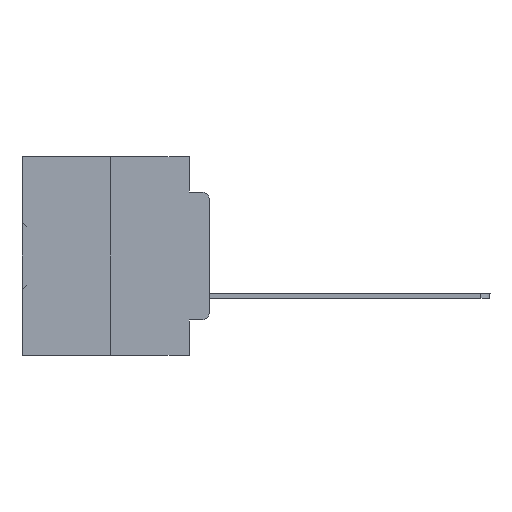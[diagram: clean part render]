
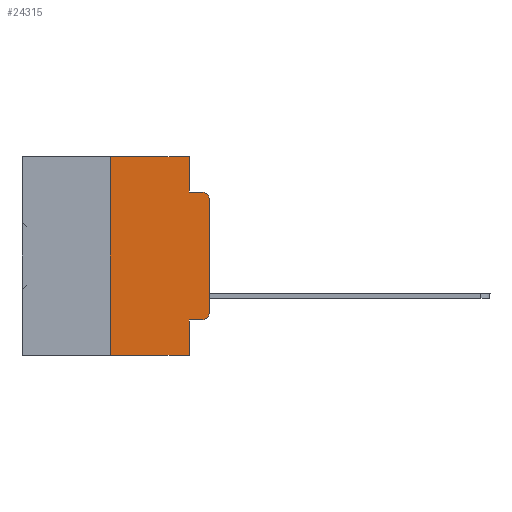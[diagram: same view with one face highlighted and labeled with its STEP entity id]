
A CAD part, left-side view. The second image highlights one B-rep face of the part: STEP entity #24315.
In plain terms, the highlighted planar face has unit normal (-1, 0, 0).
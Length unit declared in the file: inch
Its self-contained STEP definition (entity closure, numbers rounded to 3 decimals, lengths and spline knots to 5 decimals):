
#2049 = LINE ( 'NONE', #13512, #25547 ) ;
#2791 = VERTEX_POINT ( 'NONE', #32330 ) ;
#2859 = VERTEX_POINT ( 'NONE', #7158 ) ;
#3411 = EDGE_CURVE ( 'NONE', #18733, #25055, #25482, .T. ) ;
#3481 = ORIENTED_EDGE ( 'NONE', *, *, #14463, .T. ) ;
#5151 = DIRECTION ( 'NONE',  ( -1., 0., 0. ) ) ;
#5340 = VERTEX_POINT ( 'NONE', #20381 ) ;
#5866 = AXIS2_PLACEMENT_3D ( 'NONE', #30875, #5151, #28058 ) ;
#6440 = ORIENTED_EDGE ( 'NONE', *, *, #6719, .F. ) ;
#6719 = EDGE_CURVE ( 'NONE', #18733, #5340, #20243, .T. ) ;
#6981 = DIRECTION ( 'NONE',  ( 0., 0., -1. ) ) ;
#7158 = CARTESIAN_POINT ( 'NONE',  ( 0., 0.02, -0.0885 ) ) ;
#7283 = VECTOR ( 'NONE', #11411, 39.37008 ) ;
#7359 = CARTESIAN_POINT ( 'NONE',  ( 0., 0.02, -0.1085 ) ) ;
#7740 = ORIENTED_EDGE ( 'NONE', *, *, #14694, .T. ) ;
#8896 = ORIENTED_EDGE ( 'NONE', *, *, #27386, .F. ) ;
#9065 = VECTOR ( 'NONE', #19751, 39.37008 ) ;
#9411 = CARTESIAN_POINT ( 'NONE',  ( 0., 0., -0.3915 ) ) ;
#9613 = CARTESIAN_POINT ( 'NONE',  ( 0., 0.473, 0. ) ) ;
#9690 = LINE ( 'NONE', #21133, #35719 ) ;
#10529 = CIRCLE ( 'NONE', #30297, 0.02 ) ;
#10641 = EDGE_CURVE ( 'NONE', #10848, #15091, #24559, .T. ) ;
#10848 = VERTEX_POINT ( 'NONE', #17407 ) ;
#11054 = EDGE_CURVE ( 'NONE', #5340, #10848, #9690, .T. ) ;
#11411 = DIRECTION ( 'NONE',  ( 0., 0., 1. ) ) ;
#12309 = LINE ( 'NONE', #26766, #20250 ) ;
#12529 = CARTESIAN_POINT ( 'NONE',  ( 0., 0.25, -0.5 ) ) ;
#13048 = VECTOR ( 'NONE', #21058, 39.37008 ) ;
#13512 = CARTESIAN_POINT ( 'NONE',  ( 0., 0.051, -0.4115 ) ) ;
#13858 = ORIENTED_EDGE ( 'NONE', *, *, #3411, .T. ) ;
#14463 = EDGE_CURVE ( 'NONE', #37064, #36121, #12309, .T. ) ;
#14694 = EDGE_CURVE ( 'NONE', #17831, #37064, #20853, .T. ) ;
#15091 = VERTEX_POINT ( 'NONE', #19385 ) ;
#15316 = DIRECTION ( 'NONE',  ( 0., 0., 1. ) ) ;
#15439 = CARTESIAN_POINT ( 'NONE',  ( 0., 0.051, 0. ) ) ;
#16123 = DIRECTION ( 'NONE',  ( 0., 0., -1. ) ) ;
#17407 = CARTESIAN_POINT ( 'NONE',  ( 0., 0.051, 0. ) ) ;
#17831 = VERTEX_POINT ( 'NONE', #26313 ) ;
#18733 = VERTEX_POINT ( 'NONE', #12529 ) ;
#18930 = CARTESIAN_POINT ( 'NONE',  ( 0., 0.051, 0. ) ) ;
#19274 = EDGE_CURVE ( 'NONE', #15091, #2859, #32780, .T. ) ;
#19385 = CARTESIAN_POINT ( 'NONE',  ( 0., 0.051, -0.0885 ) ) ;
#19563 = CARTESIAN_POINT ( 'NONE',  ( 0., 0.051, -0.0885 ) ) ;
#19751 = DIRECTION ( 'NONE',  ( 0., -1., 0. ) ) ;
#19873 = CARTESIAN_POINT ( 'NONE',  ( 0., 0.25, 0. ) ) ;
#20198 = CARTESIAN_POINT ( 'NONE',  ( 0., 0.051, -0.5 ) ) ;
#20243 = LINE ( 'NONE', #19873, #7283 ) ;
#20250 = VECTOR ( 'NONE', #15316, 39.37008 ) ;
#20381 = CARTESIAN_POINT ( 'NONE',  ( 0., 0.25, 0. ) ) ;
#20853 = CIRCLE ( 'NONE', #5866, 0.02 ) ;
#21058 = DIRECTION ( 'NONE',  ( 0., 0., -1. ) ) ;
#21133 = CARTESIAN_POINT ( 'NONE',  ( 0., 0.473, 0. ) ) ;
#21308 = VECTOR ( 'NONE', #16123, 39.37008 ) ;
#22867 = DIRECTION ( 'NONE',  ( 0., -1., 0. ) ) ;
#22950 = ORIENTED_EDGE ( 'NONE', *, *, #11054, .F. ) ;
#24072 = ORIENTED_EDGE ( 'NONE', *, *, #33189, .T. ) ;
#24238 = PLANE ( 'NONE',  #33860 ) ;
#24240 = DIRECTION ( 'NONE',  ( -1., 0., 0. ) ) ;
#24315 = ADVANCED_FACE ( 'NONE', ( #35910 ), #24238, .F. ) ;
#24559 = LINE ( 'NONE', #18930, #21308 ) ;
#25055 = VERTEX_POINT ( 'NONE', #20198 ) ;
#25126 = DIRECTION ( 'NONE',  ( 0., -1., 0. ) ) ;
#25482 = LINE ( 'NONE', #28486, #34034 ) ;
#25547 = VECTOR ( 'NONE', #22867, 39.37008 ) ;
#26313 = CARTESIAN_POINT ( 'NONE',  ( 0., 0.02, -0.4115 ) ) ;
#26394 = CARTESIAN_POINT ( 'NONE',  ( 0., 0., -0.1085 ) ) ;
#26766 = CARTESIAN_POINT ( 'NONE',  ( 0., 0., 0. ) ) ;
#27329 = DIRECTION ( 'NONE',  ( 0., -1., 0. ) ) ;
#27386 = EDGE_CURVE ( 'NONE', #2791, #25055, #29332, .T. ) ;
#27897 = EDGE_LOOP ( 'NONE', ( #3481, #33130, #32219, #33987, #22950, #6440, #13858, #8896, #24072, #7740 ) ) ;
#28058 = DIRECTION ( 'NONE',  ( 0., 0., -1. ) ) ;
#28486 = CARTESIAN_POINT ( 'NONE',  ( 0., 0.473, -0.5 ) ) ;
#29332 = LINE ( 'NONE', #15439, #13048 ) ;
#29883 = DIRECTION ( 'NONE',  ( 1., 0., 0. ) ) ;
#30297 = AXIS2_PLACEMENT_3D ( 'NONE', #7359, #24240, #6981 ) ;
#30875 = CARTESIAN_POINT ( 'NONE',  ( 0., 0.02, -0.3915 ) ) ;
#31166 = EDGE_CURVE ( 'NONE', #36121, #2859, #10529, .T. ) ;
#32219 = ORIENTED_EDGE ( 'NONE', *, *, #19274, .F. ) ;
#32330 = CARTESIAN_POINT ( 'NONE',  ( 0., 0.051, -0.4115 ) ) ;
#32780 = LINE ( 'NONE', #19563, #9065 ) ;
#33130 = ORIENTED_EDGE ( 'NONE', *, *, #31166, .T. ) ;
#33189 = EDGE_CURVE ( 'NONE', #2791, #17831, #2049, .T. ) ;
#33860 = AXIS2_PLACEMENT_3D ( 'NONE', #9613, #29883, #35166 ) ;
#33987 = ORIENTED_EDGE ( 'NONE', *, *, #10641, .F. ) ;
#34034 = VECTOR ( 'NONE', #25126, 39.37008 ) ;
#35166 = DIRECTION ( 'NONE',  ( 0., 0., -1. ) ) ;
#35719 = VECTOR ( 'NONE', #27329, 39.37008 ) ;
#35910 = FACE_OUTER_BOUND ( 'NONE', #27897, .T. ) ;
#36121 = VERTEX_POINT ( 'NONE', #26394 ) ;
#37064 = VERTEX_POINT ( 'NONE', #9411 ) ;
